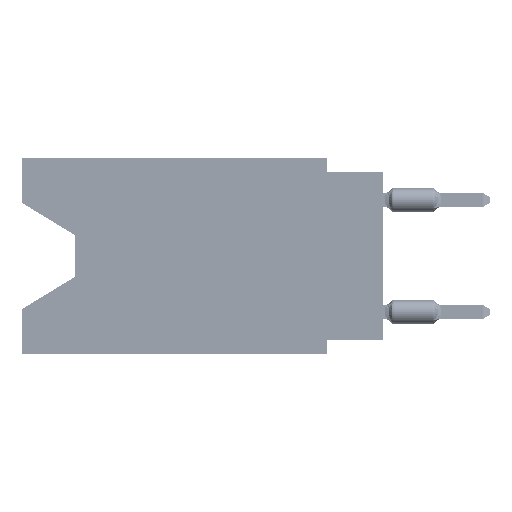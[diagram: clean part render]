
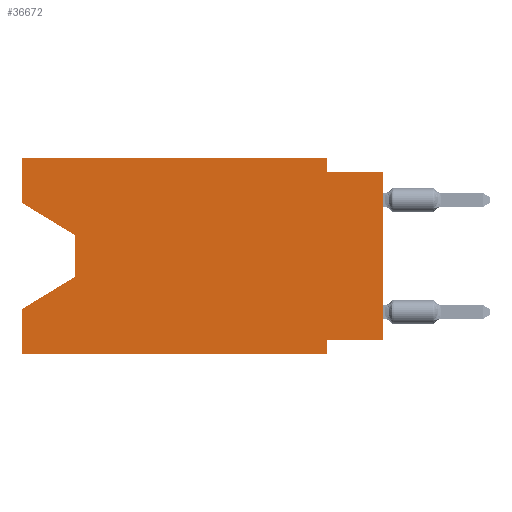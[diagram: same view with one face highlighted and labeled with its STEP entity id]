
A CAD part, left-side view. The second image highlights one B-rep face of the part: STEP entity #36672.
In plain terms, the highlighted planar face has unit normal (-1, 0, 0).
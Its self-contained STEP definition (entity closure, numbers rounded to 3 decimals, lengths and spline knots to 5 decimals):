
#990 = LINE ( 'NONE', #36281, #16065 ) ;
#1371 = VERTEX_POINT ( 'NONE', #30758 ) ;
#2849 = CARTESIAN_POINT ( 'NONE',  ( 0., 0.645, -0.35 ) ) ;
#4583 = EDGE_CURVE ( 'NONE', #112201, #97642, #38285, .T. ) ;
#6347 = VECTOR ( 'NONE', #15134, 39.37008 ) ;
#6371 = CARTESIAN_POINT ( 'NONE',  ( 0., 0.1, 0. ) ) ;
#7339 = CARTESIAN_POINT ( 'NONE',  ( 0., 0.645, 0. ) ) ;
#8190 = CARTESIAN_POINT ( 'NONE',  ( 0., 0.645, -0.08025 ) ) ;
#9385 = LINE ( 'NONE', #60626, #13548 ) ;
#9653 = CARTESIAN_POINT ( 'NONE',  ( 0., 0.55, -0.138 ) ) ;
#13282 = EDGE_CURVE ( 'NONE', #112450, #59811, #76986, .T. ) ;
#13548 = VECTOR ( 'NONE', #95338, 39.37008 ) ;
#13699 = EDGE_CURVE ( 'NONE', #59811, #53264, #91686, .T. ) ;
#13714 = DIRECTION ( 'NONE',  ( 0., 0., -1. ) ) ;
#13841 = CARTESIAN_POINT ( 'NONE',  ( 0., 0.1, 0. ) ) ;
#14274 = EDGE_CURVE ( 'NONE', #18745, #93035, #9385, .T. ) ;
#15134 = DIRECTION ( 'NONE',  ( 0., -1., 0. ) ) ;
#15555 = CARTESIAN_POINT ( 'NONE',  ( 0., 0., -0.325 ) ) ;
#16065 = VECTOR ( 'NONE', #51663, 39.37008 ) ;
#17301 = CARTESIAN_POINT ( 'NONE',  ( 0., 0.645, -0.26975 ) ) ;
#18745 = VERTEX_POINT ( 'NONE', #2849 ) ;
#19041 = AXIS2_PLACEMENT_3D ( 'NONE', #111006, #60362, #95064 ) ;
#19131 = ORIENTED_EDGE ( 'NONE', *, *, #61766, .T. ) ;
#19251 = DIRECTION ( 'NONE',  ( 0., 0.855, -0.519 ) ) ;
#22042 = EDGE_CURVE ( 'NONE', #53264, #93035, #79587, .T. ) ;
#22622 = VECTOR ( 'NONE', #107147, 39.37008 ) ;
#23750 = VECTOR ( 'NONE', #91810, 39.37008 ) ;
#23979 = EDGE_CURVE ( 'NONE', #54879, #1371, #990, .T. ) ;
#25858 = DIRECTION ( 'NONE',  ( 0., -1., 0. ) ) ;
#27235 = ORIENTED_EDGE ( 'NONE', *, *, #38113, .F. ) ;
#28914 = ORIENTED_EDGE ( 'NONE', *, *, #47475, .F. ) ;
#29730 = VECTOR ( 'NONE', #67882, 39.37008 ) ;
#30295 = VECTOR ( 'NONE', #32575, 39.37008 ) ;
#30758 = CARTESIAN_POINT ( 'NONE',  ( 0., 0., -0.025 ) ) ;
#32050 = LINE ( 'NONE', #13841, #23750 ) ;
#32575 = DIRECTION ( 'NONE',  ( 0., 0., -1. ) ) ;
#35579 = VERTEX_POINT ( 'NONE', #48290 ) ;
#36281 = CARTESIAN_POINT ( 'NONE',  ( 0., 0., 0. ) ) ;
#36672 = ADVANCED_FACE ( 'NONE', ( #104171 ), #85396, .F. ) ;
#37113 = VERTEX_POINT ( 'NONE', #50564 ) ;
#38113 = EDGE_CURVE ( 'NONE', #54879, #35579, #51994, .T. ) ;
#38285 = LINE ( 'NONE', #88404, #22622 ) ;
#39534 = ORIENTED_EDGE ( 'NONE', *, *, #94647, .F. ) ;
#41259 = VECTOR ( 'NONE', #19251, 39.37008 ) ;
#41868 = LINE ( 'NONE', #66947, #6347 ) ;
#44642 = CARTESIAN_POINT ( 'NONE',  ( 0., 0., -0.025 ) ) ;
#46653 = DIRECTION ( 'NONE',  ( 0., 1., 0. ) ) ;
#47475 = EDGE_CURVE ( 'NONE', #37113, #1371, #60017, .T. ) ;
#48290 = CARTESIAN_POINT ( 'NONE',  ( 0., 0.1, -0.325 ) ) ;
#50564 = CARTESIAN_POINT ( 'NONE',  ( 0., 0.1, -0.025 ) ) ;
#51663 = DIRECTION ( 'NONE',  ( 0., 0., 1. ) ) ;
#51994 = LINE ( 'NONE', #90459, #88413 ) ;
#53247 = VECTOR ( 'NONE', #25858, 39.37008 ) ;
#53264 = VERTEX_POINT ( 'NONE', #92532 ) ;
#54879 = VERTEX_POINT ( 'NONE', #15555 ) ;
#57291 = ORIENTED_EDGE ( 'NONE', *, *, #22042, .T. ) ;
#59811 = VERTEX_POINT ( 'NONE', #9653 ) ;
#60017 = LINE ( 'NONE', #44642, #53247 ) ;
#60362 = DIRECTION ( 'NONE',  ( 1., 0., 0. ) ) ;
#60626 = CARTESIAN_POINT ( 'NONE',  ( 0., 0.645, 0. ) ) ;
#60691 = VECTOR ( 'NONE', #13714, 39.37008 ) ;
#61045 = ORIENTED_EDGE ( 'NONE', *, *, #14274, .F. ) ;
#61766 = EDGE_CURVE ( 'NONE', #18745, #110525, #41868, .T. ) ;
#63545 = ORIENTED_EDGE ( 'NONE', *, *, #13699, .T. ) ;
#66947 = CARTESIAN_POINT ( 'NONE',  ( 0., 0.645, -0.35 ) ) ;
#67882 = DIRECTION ( 'NONE',  ( 0., -0.855, -0.519 ) ) ;
#75261 = DIRECTION ( 'NONE',  ( 0., 0., 1. ) ) ;
#76986 = LINE ( 'NONE', #92925, #29730 ) ;
#78921 = ORIENTED_EDGE ( 'NONE', *, *, #102127, .F. ) ;
#79587 = LINE ( 'NONE', #80695, #41259 ) ;
#80695 = CARTESIAN_POINT ( 'NONE',  ( 0., 0.55, -0.212 ) ) ;
#80701 = ORIENTED_EDGE ( 'NONE', *, *, #23979, .T. ) ;
#83780 = LINE ( 'NONE', #110521, #86833 ) ;
#85025 = ORIENTED_EDGE ( 'NONE', *, *, #4583, .F. ) ;
#85396 = PLANE ( 'NONE',  #19041 ) ;
#85472 = CARTESIAN_POINT ( 'NONE',  ( 0., 0.1, -0.35 ) ) ;
#86833 = VECTOR ( 'NONE', #75261, 39.37008 ) ;
#88404 = CARTESIAN_POINT ( 'NONE',  ( 0., 0.645, 0. ) ) ;
#88413 = VECTOR ( 'NONE', #46653, 39.37008 ) ;
#89011 = CARTESIAN_POINT ( 'NONE',  ( 0., 0.1, -0.35 ) ) ;
#90459 = CARTESIAN_POINT ( 'NONE',  ( 0., 0., -0.325 ) ) ;
#91325 = EDGE_LOOP ( 'NONE', ( #94237, #63545, #57291, #61045, #19131, #39534, #27235, #80701, #28914, #78921, #85025, #93136 ) ) ;
#91686 = LINE ( 'NONE', #103436, #60691 ) ;
#91810 = DIRECTION ( 'NONE',  ( 0., 0., -1. ) ) ;
#92532 = CARTESIAN_POINT ( 'NONE',  ( 0., 0.55, -0.212 ) ) ;
#92925 = CARTESIAN_POINT ( 'NONE',  ( 0., 0.645, -0.08025 ) ) ;
#93035 = VERTEX_POINT ( 'NONE', #17301 ) ;
#93136 = ORIENTED_EDGE ( 'NONE', *, *, #97686, .F. ) ;
#94237 = ORIENTED_EDGE ( 'NONE', *, *, #13282, .T. ) ;
#94647 = EDGE_CURVE ( 'NONE', #35579, #110525, #110537, .T. ) ;
#95064 = DIRECTION ( 'NONE',  ( 0., 0., -1. ) ) ;
#95338 = DIRECTION ( 'NONE',  ( 0., 0., 1. ) ) ;
#97642 = VERTEX_POINT ( 'NONE', #6371 ) ;
#97686 = EDGE_CURVE ( 'NONE', #112450, #112201, #83780, .T. ) ;
#102127 = EDGE_CURVE ( 'NONE', #97642, #37113, #32050, .T. ) ;
#103436 = CARTESIAN_POINT ( 'NONE',  ( 0., 0.55, -0.138 ) ) ;
#104171 = FACE_OUTER_BOUND ( 'NONE', #91325, .T. ) ;
#107147 = DIRECTION ( 'NONE',  ( 0., -1., 0. ) ) ;
#110521 = CARTESIAN_POINT ( 'NONE',  ( 0., 0.645, 0. ) ) ;
#110525 = VERTEX_POINT ( 'NONE', #89011 ) ;
#110537 = LINE ( 'NONE', #85472, #30295 ) ;
#111006 = CARTESIAN_POINT ( 'NONE',  ( 0., 0.645, 0. ) ) ;
#112201 = VERTEX_POINT ( 'NONE', #7339 ) ;
#112450 = VERTEX_POINT ( 'NONE', #8190 ) ;
